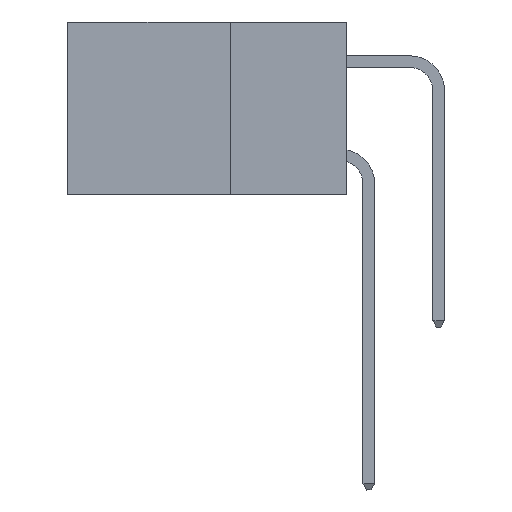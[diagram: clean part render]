
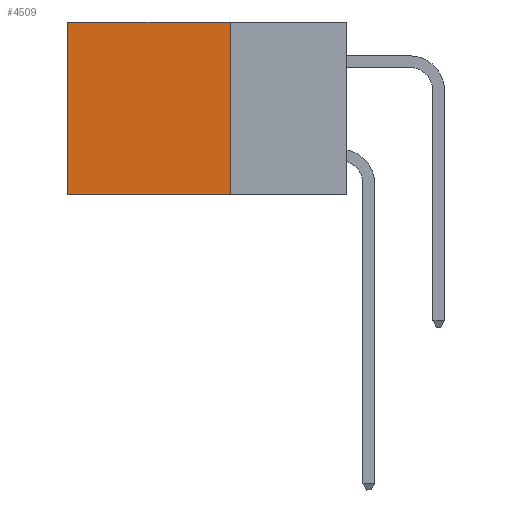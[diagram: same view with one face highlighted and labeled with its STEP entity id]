
A CAD part, left-side view. The second image highlights one B-rep face of the part: STEP entity #4509.
In plain terms, the highlighted planar face has unit normal (-1, 0, 0).
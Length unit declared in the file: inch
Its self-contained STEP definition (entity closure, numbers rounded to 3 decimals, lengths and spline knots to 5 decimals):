
#337 = CARTESIAN_POINT ( 'NONE',  ( 0.2875, 0.6, 0. ) ) ;
#709 = CARTESIAN_POINT ( 'NONE',  ( 0.2875, 0.25, 0. ) ) ;
#1665 = DIRECTION ( 'NONE',  ( 0., 0., -1. ) ) ;
#1811 = AXIS2_PLACEMENT_3D ( 'NONE', #11187, #16919, #17100 ) ;
#3007 = LINE ( 'NONE', #21882, #17511 ) ;
#3274 = ORIENTED_EDGE ( 'NONE', *, *, #10538, .T. ) ;
#3356 = EDGE_CURVE ( 'NONE', #22303, #7240, #3007, .T. ) ;
#4509 = ADVANCED_FACE ( 'NONE', ( #20185 ), #17280, .F. ) ;
#6156 = CARTESIAN_POINT ( 'NONE',  ( 0.2875, 0.25, 0. ) ) ;
#6912 = ORIENTED_EDGE ( 'NONE', *, *, #24110, .T. ) ;
#7240 = VERTEX_POINT ( 'NONE', #8542 ) ;
#8542 = CARTESIAN_POINT ( 'NONE',  ( 0.2875, 0.6, -0.37 ) ) ;
#9187 = VERTEX_POINT ( 'NONE', #21553 ) ;
#9884 = VECTOR ( 'NONE', #10501, 39.37008 ) ;
#10501 = DIRECTION ( 'NONE',  ( 0., 0., -1. ) ) ;
#10538 = EDGE_CURVE ( 'NONE', #9187, #7240, #14579, .T. ) ;
#10872 = VECTOR ( 'NONE', #1665, 39.37008 ) ;
#11187 = CARTESIAN_POINT ( 'NONE',  ( 0.2875, 0.25, 0. ) ) ;
#11517 = CARTESIAN_POINT ( 'NONE',  ( 0.2875, 0.25, 0. ) ) ;
#12839 = VERTEX_POINT ( 'NONE', #6156 ) ;
#12842 = DIRECTION ( 'NONE',  ( 0., 1., 0. ) ) ;
#13495 = DIRECTION ( 'NONE',  ( 0., 1., 0. ) ) ;
#14579 = LINE ( 'NONE', #337, #9884 ) ;
#16919 = DIRECTION ( 'NONE',  ( 1., 0., 0. ) ) ;
#17100 = DIRECTION ( 'NONE',  ( 0., 0., -1. ) ) ;
#17130 = CARTESIAN_POINT ( 'NONE',  ( 0.2875, 0.25, -0.37 ) ) ;
#17280 = PLANE ( 'NONE',  #1811 ) ;
#17511 = VECTOR ( 'NONE', #13495, 39.37008 ) ;
#17722 = ORIENTED_EDGE ( 'NONE', *, *, #24964, .F. ) ;
#18456 = LINE ( 'NONE', #11517, #10872 ) ;
#19128 = VECTOR ( 'NONE', #12842, 39.37008 ) ;
#20185 = FACE_OUTER_BOUND ( 'NONE', #20968, .T. ) ;
#20968 = EDGE_LOOP ( 'NONE', ( #3274, #23255, #17722, #6912 ) ) ;
#21553 = CARTESIAN_POINT ( 'NONE',  ( 0.2875, 0.6, 0. ) ) ;
#21882 = CARTESIAN_POINT ( 'NONE',  ( 0.2875, 0.25, -0.37 ) ) ;
#22303 = VERTEX_POINT ( 'NONE', #17130 ) ;
#23255 = ORIENTED_EDGE ( 'NONE', *, *, #3356, .F. ) ;
#24110 = EDGE_CURVE ( 'NONE', #12839, #9187, #24465, .T. ) ;
#24465 = LINE ( 'NONE', #709, #19128 ) ;
#24964 = EDGE_CURVE ( 'NONE', #12839, #22303, #18456, .T. ) ;
